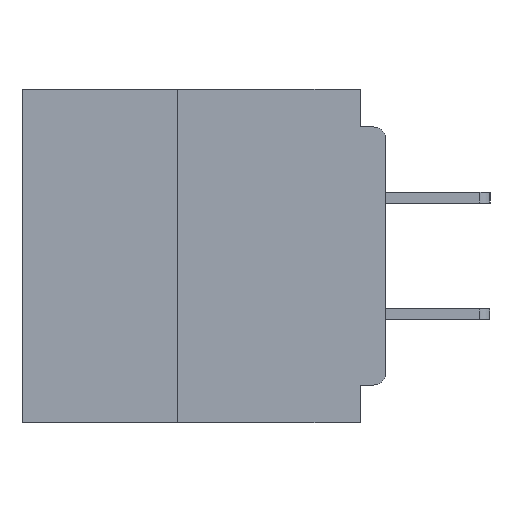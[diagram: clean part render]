
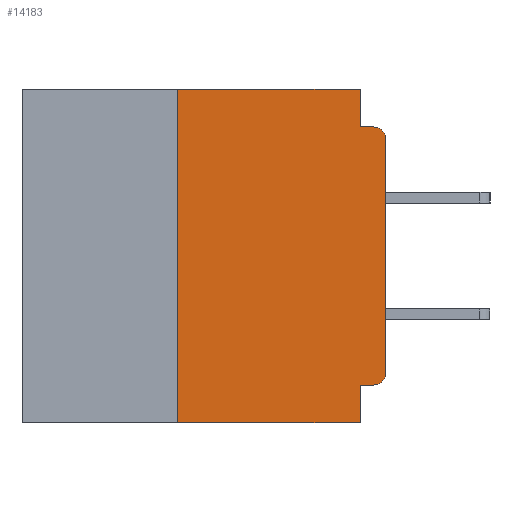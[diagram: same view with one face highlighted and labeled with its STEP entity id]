
A CAD part, left-side view. The second image highlights one B-rep face of the part: STEP entity #14183.
In plain terms, the highlighted planar face has unit normal (-1, 0, 0).
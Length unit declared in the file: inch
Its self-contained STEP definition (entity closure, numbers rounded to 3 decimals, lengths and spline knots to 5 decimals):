
#116 = ORIENTED_EDGE ( 'NONE', *, *, #20042, .T. ) ;
#1349 = VERTEX_POINT ( 'NONE', #47390 ) ;
#4104 = DIRECTION ( 'NONE',  ( 1., 0., 0. ) ) ;
#4628 = DIRECTION ( 'NONE',  ( 0., -1., 0. ) ) ;
#6242 = CARTESIAN_POINT ( 'NONE',  ( 0., 0.25, -0.4 ) ) ;
#7204 = CARTESIAN_POINT ( 'NONE',  ( 0., 0., -0.045 ) ) ;
#9120 = DIRECTION ( 'NONE',  ( 0., 0., 1. ) ) ;
#9547 = AXIS2_PLACEMENT_3D ( 'NONE', #12654, #4104, #21226 ) ;
#10419 = CARTESIAN_POINT ( 'NONE',  ( 0., 0.015, -0.34 ) ) ;
#10790 = VERTEX_POINT ( 'NONE', #12722 ) ;
#12474 = AXIS2_PLACEMENT_3D ( 'NONE', #10419, #39857, #14721 ) ;
#12654 = CARTESIAN_POINT ( 'NONE',  ( 0., 0.437, 0. ) ) ;
#12657 = CARTESIAN_POINT ( 'NONE',  ( 0., 0., -0.06 ) ) ;
#12722 = CARTESIAN_POINT ( 'NONE',  ( 0., 0., -0.34 ) ) ;
#13454 = CARTESIAN_POINT ( 'NONE',  ( 0., 0.25, -0.4 ) ) ;
#13461 = ORIENTED_EDGE ( 'NONE', *, *, #14316, .F. ) ;
#14032 = LINE ( 'NONE', #13454, #46018 ) ;
#14183 = ADVANCED_FACE ( 'NONE', ( #38517 ), #16949, .F. ) ;
#14316 = EDGE_CURVE ( 'NONE', #44124, #28752, #42999, .T. ) ;
#14549 = LINE ( 'NONE', #27061, #35577 ) ;
#14721 = DIRECTION ( 'NONE',  ( 0., 0., -1. ) ) ;
#15312 = VECTOR ( 'NONE', #31010, 39.37008 ) ;
#15797 = EDGE_CURVE ( 'NONE', #53649, #1349, #25960, .T. ) ;
#16501 = EDGE_CURVE ( 'NONE', #33283, #53649, #14032, .T. ) ;
#16949 = PLANE ( 'NONE',  #9547 ) ;
#17272 = VECTOR ( 'NONE', #4628, 39.37008 ) ;
#17499 = CARTESIAN_POINT ( 'NONE',  ( 0., 0.437, -0.4 ) ) ;
#17798 = CIRCLE ( 'NONE', #12474, 0.015 ) ;
#18108 = ORIENTED_EDGE ( 'NONE', *, *, #16501, .F. ) ;
#19484 = VERTEX_POINT ( 'NONE', #53392 ) ;
#20042 = EDGE_CURVE ( 'NONE', #38769, #33221, #36479, .T. ) ;
#20864 = VECTOR ( 'NONE', #50841, 39.37008 ) ;
#21226 = DIRECTION ( 'NONE',  ( 0., 0., -1. ) ) ;
#21281 = LINE ( 'NONE', #46082, #42133 ) ;
#21413 = VECTOR ( 'NONE', #52950, 39.37008 ) ;
#22124 = EDGE_CURVE ( 'NONE', #10790, #38769, #21281, .T. ) ;
#22200 = EDGE_CURVE ( 'NONE', #33283, #24535, #50364, .T. ) ;
#22736 = ORIENTED_EDGE ( 'NONE', *, *, #26618, .F. ) ;
#24164 = DIRECTION ( 'NONE',  ( -1., 0., 0. ) ) ;
#24535 = VERTEX_POINT ( 'NONE', #38900 ) ;
#25318 = ORIENTED_EDGE ( 'NONE', *, *, #50915, .F. ) ;
#25960 = LINE ( 'NONE', #50436, #35811 ) ;
#26618 = EDGE_CURVE ( 'NONE', #19484, #33221, #44817, .T. ) ;
#26632 = EDGE_LOOP ( 'NONE', ( #32490, #116, #22736, #25318, #47366, #18108, #41675, #34516, #13461, #48025 ) ) ;
#26800 = CARTESIAN_POINT ( 'NONE',  ( 0., 0.031, 0. ) ) ;
#27061 = CARTESIAN_POINT ( 'NONE',  ( 0., 0.031, -0.4 ) ) ;
#28752 = VERTEX_POINT ( 'NONE', #49074 ) ;
#30110 = CARTESIAN_POINT ( 'NONE',  ( 0., 0., -0.355 ) ) ;
#31010 = DIRECTION ( 'NONE',  ( 0., 0., -1. ) ) ;
#32490 = ORIENTED_EDGE ( 'NONE', *, *, #22124, .T. ) ;
#33221 = VERTEX_POINT ( 'NONE', #39579 ) ;
#33283 = VERTEX_POINT ( 'NONE', #6242 ) ;
#34516 = ORIENTED_EDGE ( 'NONE', *, *, #38973, .F. ) ;
#35577 = VECTOR ( 'NONE', #39730, 39.37008 ) ;
#35811 = VECTOR ( 'NONE', #38141, 39.37008 ) ;
#36479 = CIRCLE ( 'NONE', #52049, 0.015 ) ;
#37631 = LINE ( 'NONE', #26800, #15312 ) ;
#37849 = DIRECTION ( 'NONE',  ( 0., 0., 1. ) ) ;
#38141 = DIRECTION ( 'NONE',  ( 0., -1., 0. ) ) ;
#38517 = FACE_OUTER_BOUND ( 'NONE', #26632, .T. ) ;
#38769 = VERTEX_POINT ( 'NONE', #12657 ) ;
#38900 = CARTESIAN_POINT ( 'NONE',  ( 0., 0.031, -0.4 ) ) ;
#38973 = EDGE_CURVE ( 'NONE', #28752, #24535, #14549, .T. ) ;
#39579 = CARTESIAN_POINT ( 'NONE',  ( 0., 0.015, -0.045 ) ) ;
#39616 = EDGE_CURVE ( 'NONE', #44124, #10790, #17798, .T. ) ;
#39730 = DIRECTION ( 'NONE',  ( 0., 0., -1. ) ) ;
#39857 = DIRECTION ( 'NONE',  ( -1., 0., 0. ) ) ;
#41675 = ORIENTED_EDGE ( 'NONE', *, *, #22200, .T. ) ;
#41906 = CARTESIAN_POINT ( 'NONE',  ( 0., 0.015, -0.355 ) ) ;
#42133 = VECTOR ( 'NONE', #37849, 39.37008 ) ;
#42907 = CARTESIAN_POINT ( 'NONE',  ( 0., 0.25, 0. ) ) ;
#42999 = LINE ( 'NONE', #30110, #20864 ) ;
#44124 = VERTEX_POINT ( 'NONE', #41906 ) ;
#44817 = LINE ( 'NONE', #7204, #21413 ) ;
#46018 = VECTOR ( 'NONE', #9120, 39.37008 ) ;
#46082 = CARTESIAN_POINT ( 'NONE',  ( 0., 0., 0. ) ) ;
#47366 = ORIENTED_EDGE ( 'NONE', *, *, #15797, .F. ) ;
#47390 = CARTESIAN_POINT ( 'NONE',  ( 0., 0.031, 0. ) ) ;
#48025 = ORIENTED_EDGE ( 'NONE', *, *, #39616, .T. ) ;
#48944 = CARTESIAN_POINT ( 'NONE',  ( 0., 0.015, -0.06 ) ) ;
#49074 = CARTESIAN_POINT ( 'NONE',  ( 0., 0.031, -0.355 ) ) ;
#50364 = LINE ( 'NONE', #17499, #17272 ) ;
#50436 = CARTESIAN_POINT ( 'NONE',  ( 0., 0.437, 0. ) ) ;
#50841 = DIRECTION ( 'NONE',  ( 0., 1., 0. ) ) ;
#50915 = EDGE_CURVE ( 'NONE', #1349, #19484, #37631, .T. ) ;
#52049 = AXIS2_PLACEMENT_3D ( 'NONE', #48944, #24164, #52997 ) ;
#52950 = DIRECTION ( 'NONE',  ( 0., -1., 0. ) ) ;
#52997 = DIRECTION ( 'NONE',  ( 0., 0., -1. ) ) ;
#53392 = CARTESIAN_POINT ( 'NONE',  ( 0., 0.031, -0.045 ) ) ;
#53649 = VERTEX_POINT ( 'NONE', #42907 ) ;
